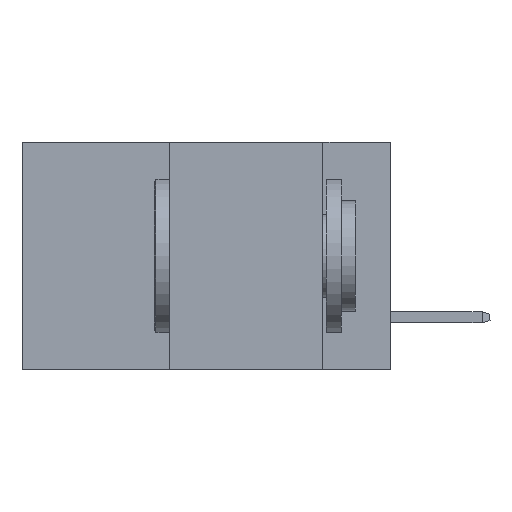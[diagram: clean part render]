
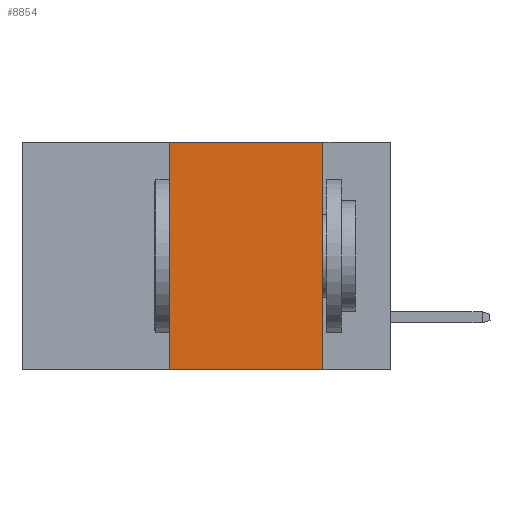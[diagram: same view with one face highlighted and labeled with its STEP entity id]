
A CAD part, left-side view. The second image highlights one B-rep face of the part: STEP entity #8854.
In plain terms, the highlighted planar face has unit normal (-1, 0, 0).
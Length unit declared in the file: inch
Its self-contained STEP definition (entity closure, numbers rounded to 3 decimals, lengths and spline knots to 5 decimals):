
#86 = EDGE_LOOP ( 'NONE', ( #9471, #7426, #2940, #11665 ) ) ;
#1360 = VERTEX_POINT ( 'NONE', #8378 ) ;
#1475 = VECTOR ( 'NONE', #10769, 39.37008 ) ;
#1740 = CARTESIAN_POINT ( 'NONE',  ( 0., 0.11, 0. ) ) ;
#2281 = DIRECTION ( 'NONE',  ( 0., 0., -1. ) ) ;
#2311 = FACE_OUTER_BOUND ( 'NONE', #86, .T. ) ;
#2506 = CARTESIAN_POINT ( 'NONE',  ( 0., 0.11, 0. ) ) ;
#2687 = DIRECTION ( 'NONE',  ( 0., 0., -1. ) ) ;
#2770 = LINE ( 'NONE', #2506, #9925 ) ;
#2940 = ORIENTED_EDGE ( 'NONE', *, *, #12992, .F. ) ;
#3954 = DIRECTION ( 'NONE',  ( 0., -1., 0. ) ) ;
#4075 = EDGE_CURVE ( 'NONE', #11448, #10967, #2770, .T. ) ;
#4173 = VERTEX_POINT ( 'NONE', #10123 ) ;
#4547 = LINE ( 'NONE', #11738, #1475 ) ;
#5204 = LINE ( 'NONE', #11746, #10252 ) ;
#7426 = ORIENTED_EDGE ( 'NONE', *, *, #10597, .F. ) ;
#7622 = VECTOR ( 'NONE', #3954, 39.37008 ) ;
#7915 = LINE ( 'NONE', #10032, #7622 ) ;
#8378 = CARTESIAN_POINT ( 'NONE',  ( 0., 0.36, -0.37 ) ) ;
#8390 = DIRECTION ( 'NONE',  ( 1., 0., 0. ) ) ;
#8538 = CARTESIAN_POINT ( 'NONE',  ( 0., 0.11, -0.37 ) ) ;
#8854 = ADVANCED_FACE ( 'NONE', ( #2311 ), #12375, .F. ) ;
#9471 = ORIENTED_EDGE ( 'NONE', *, *, #4075, .F. ) ;
#9830 = EDGE_CURVE ( 'NONE', #1360, #10967, #5204, .T. ) ;
#9925 = VECTOR ( 'NONE', #2687, 39.37008 ) ;
#10032 = CARTESIAN_POINT ( 'NONE',  ( 0., 0.6, 0. ) ) ;
#10123 = CARTESIAN_POINT ( 'NONE',  ( 0., 0.36, 0. ) ) ;
#10231 = AXIS2_PLACEMENT_3D ( 'NONE', #10363, #8390, #2281 ) ;
#10252 = VECTOR ( 'NONE', #12735, 39.37008 ) ;
#10363 = CARTESIAN_POINT ( 'NONE',  ( 0., 0.6, 0. ) ) ;
#10597 = EDGE_CURVE ( 'NONE', #4173, #11448, #7915, .T. ) ;
#10769 = DIRECTION ( 'NONE',  ( 0., 0., 1. ) ) ;
#10967 = VERTEX_POINT ( 'NONE', #8538 ) ;
#11448 = VERTEX_POINT ( 'NONE', #1740 ) ;
#11665 = ORIENTED_EDGE ( 'NONE', *, *, #9830, .T. ) ;
#11738 = CARTESIAN_POINT ( 'NONE',  ( 0., 0.36, 0. ) ) ;
#11746 = CARTESIAN_POINT ( 'NONE',  ( 0., 0.6, -0.37 ) ) ;
#12375 = PLANE ( 'NONE',  #10231 ) ;
#12735 = DIRECTION ( 'NONE',  ( 0., -1., 0. ) ) ;
#12992 = EDGE_CURVE ( 'NONE', #1360, #4173, #4547, .T. ) ;
